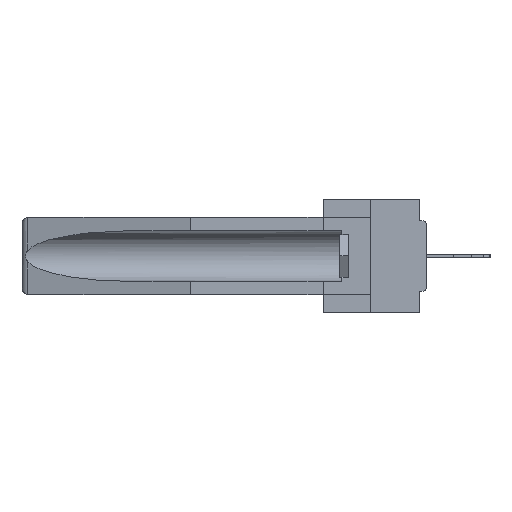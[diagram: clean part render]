
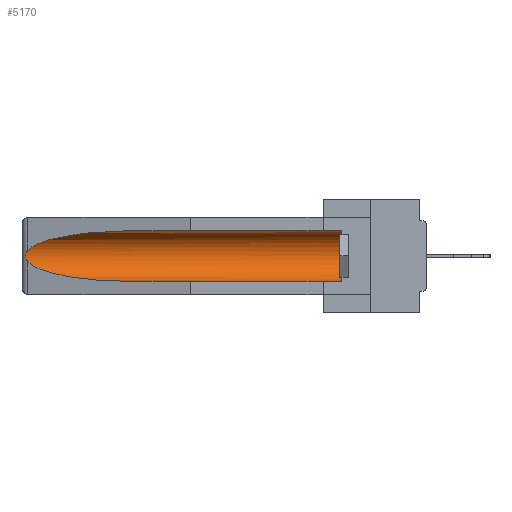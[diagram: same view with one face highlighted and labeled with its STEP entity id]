
A CAD part, left-side view. The second image highlights one B-rep face of the part: STEP entity #5170.
In plain terms, the highlighted cylindrical face has radius 2.857 mm (diameter 5.715 mm), a partial arc.
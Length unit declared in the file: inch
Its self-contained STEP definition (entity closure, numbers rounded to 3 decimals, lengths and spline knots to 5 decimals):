
#33 = CARTESIAN_POINT ( 'NONE',  ( 0.26537, 1.52718, -0.14972 ) ) ;
#827 = CARTESIAN_POINT ( 'NONE',  ( 0.25451, 1.48313, -0.09465 ) ) ;
#1087 = CARTESIAN_POINT ( 'NONE',  ( 0.25451, 1.48313, -0.24835 ) ) ;
#1258 = CARTESIAN_POINT ( 'NONE',  ( 0.21114, 1.30732, -0.284 ) ) ;
#2369 = CARTESIAN_POINT ( 'NONE',  ( 0.26597, 1.5296, -0.19026 ) ) ;
#2373 = DIRECTION ( 'NONE',  ( 0., -1., 0. ) ) ;
#3196 = VERTEX_POINT ( 'NONE', #5881 ) ;
#3373 = CARTESIAN_POINT ( 'NONE',  ( 0.155, 0.126, -0.284 ) ) ;
#4518 = CYLINDRICAL_SURFACE ( 'NONE', #18941, 0.1125 ) ;
#4991 = CARTESIAN_POINT ( 'NONE',  ( 0.26654, 1.53092, -0.15636 ) ) ;
#5170 = ADVANCED_FACE ( 'NONE', ( #16245 ), #4518, .F. ) ;
#5672 = DIRECTION ( 'NONE',  ( 0., 1., 0. ) ) ;
#5881 = CARTESIAN_POINT ( 'NONE',  ( 0.155, 1.07973, -0.059 ) ) ;
#5895 = ORIENTED_EDGE ( 'NONE', *, *, #28926, .T. ) ;
#5898 = VERTEX_POINT ( 'NONE', #27135 ) ;
#5992 =( BOUNDED_CURVE ( )  B_SPLINE_CURVE ( 3, ( #6052, #1087, #1258, #17963 ),
 .UNSPECIFIED., .F., .F. ) 
 B_SPLINE_CURVE_WITH_KNOTS ( ( 4, 4 ),
 ( 0.1948, 1.5708 ),
 .UNSPECIFIED. ) 
 CURVE ( )  GEOMETRIC_REPRESENTATION_ITEM ( )  RATIONAL_B_SPLINE_CURVE ( ( 1., 0.848, 0.848, 1. ) ) 
 REPRESENTATION_ITEM ( '' )  );
#6052 = CARTESIAN_POINT ( 'NONE',  ( 0.26537, 1.52718, -0.19328 ) ) ;
#9015 = ORIENTED_EDGE ( 'NONE', *, *, #17161, .F. ) ;
#9299 = DIRECTION ( 'NONE',  ( 0., 0., 1. ) ) ;
#10265 = CARTESIAN_POINT ( 'NONE',  ( 0.155, 1.07973, -0.059 ) ) ;
#11340 = CARTESIAN_POINT ( 'NONE',  ( 0.26537, 1.52718, -0.19328 ) ) ;
#11506 = ORIENTED_EDGE ( 'NONE', *, *, #30200, .T. ) ;
#11618 = DIRECTION ( 'NONE',  ( 0., 1., 0. ) ) ;
#11754 = LINE ( 'NONE', #25484, #19758 ) ;
#13215 = CARTESIAN_POINT ( 'NONE',  ( 0.26537, 1.52718, -0.14972 ) ) ;
#13261 = ORIENTED_EDGE ( 'NONE', *, *, #29223, .T. ) ;
#13619 = AXIS2_PLACEMENT_3D ( 'NONE', #18753, #2373, #28295 ) ;
#14417 = CARTESIAN_POINT ( 'NONE',  ( 0.26537, 1.52718, -0.19328 ) ) ;
#14434 = CARTESIAN_POINT ( 'NONE',  ( 0.2675, 1.53308, -0.17534 ) ) ;
#14921 = CARTESIAN_POINT ( 'NONE',  ( 0.26537, 1.52718, -0.14972 ) ) ;
#15838 = ORIENTED_EDGE ( 'NONE', *, *, #17611, .T. ) ;
#16245 = FACE_OUTER_BOUND ( 'NONE', #21789, .T. ) ;
#16270 = CARTESIAN_POINT ( 'NONE',  ( 0.2675, 1.53308, -0.16763 ) ) ;
#16675 = DIRECTION ( 'NONE',  ( 0., 1., 0. ) ) ;
#16735 = VERTEX_POINT ( 'NONE', #3373 ) ;
#16794 = B_SPLINE_CURVE_WITH_KNOTS ( 'NONE', 3,
 ( #33, #26119, #4991, #30167, #16270, #14434, #23837, #21062, #2369, #11340 ),
 .UNSPECIFIED., .F., .F.,
 ( 4, 2, 2, 2, 4 ),
 ( 0., 0.00029, 0.00058, 0.00087, 0.00117 ),
 .UNSPECIFIED. ) ;
#17161 = EDGE_CURVE ( 'NONE', #16735, #29163, #24661, .T. ) ;
#17611 = EDGE_CURVE ( 'NONE', #3196, #22894, #25350, .T. ) ;
#17963 = CARTESIAN_POINT ( 'NONE',  ( 0.155, 1.07973, -0.284 ) ) ;
#18753 = CARTESIAN_POINT ( 'NONE',  ( 0.155, 0.126, -0.1715 ) ) ;
#18941 = AXIS2_PLACEMENT_3D ( 'NONE', #23363, #11618, #9299 ) ;
#19545 = CARTESIAN_POINT ( 'NONE',  ( 0.21114, 1.30732, -0.059 ) ) ;
#19588 = VERTEX_POINT ( 'NONE', #14417 ) ;
#19722 = CARTESIAN_POINT ( 'NONE',  ( 0.155, -0.30754, -0.284 ) ) ;
#19758 = VECTOR ( 'NONE', #16675, 39.37008 ) ;
#21034 = ORIENTED_EDGE ( 'NONE', *, *, #25927, .T. ) ;
#21062 = CARTESIAN_POINT ( 'NONE',  ( 0.26655, 1.53094, -0.18657 ) ) ;
#21789 = EDGE_LOOP ( 'NONE', ( #15838, #5895, #13261, #9015, #11506, #21034 ) ) ;
#22894 = VERTEX_POINT ( 'NONE', #13215 ) ;
#23363 = CARTESIAN_POINT ( 'NONE',  ( 0.155, -0.30754, -0.1715 ) ) ;
#23837 = CARTESIAN_POINT ( 'NONE',  ( 0.2673, 1.53269, -0.17917 ) ) ;
#24407 = VECTOR ( 'NONE', #5672, 39.37008 ) ;
#24661 = LINE ( 'NONE', #19722, #24407 ) ;
#25042 = CARTESIAN_POINT ( 'NONE',  ( 0.155, 1.07973, -0.284 ) ) ;
#25350 =( BOUNDED_CURVE ( )  B_SPLINE_CURVE ( 3, ( #10265, #19545, #827, #14921 ),
 .UNSPECIFIED., .F., .F. ) 
 B_SPLINE_CURVE_WITH_KNOTS ( ( 4, 4 ),
 ( 4.71239, 6.08839 ),
 .UNSPECIFIED. ) 
 CURVE ( )  GEOMETRIC_REPRESENTATION_ITEM ( )  RATIONAL_B_SPLINE_CURVE ( ( 1., 0.848, 0.848, 1. ) ) 
 REPRESENTATION_ITEM ( '' )  );
#25484 = CARTESIAN_POINT ( 'NONE',  ( 0.155, -0.30754, -0.059 ) ) ;
#25927 = EDGE_CURVE ( 'NONE', #5898, #3196, #11754, .T. ) ;
#26119 = CARTESIAN_POINT ( 'NONE',  ( 0.26597, 1.52961, -0.15275 ) ) ;
#27135 = CARTESIAN_POINT ( 'NONE',  ( 0.155, 0.126, -0.059 ) ) ;
#28295 = DIRECTION ( 'NONE',  ( 0., 0., 1. ) ) ;
#28926 = EDGE_CURVE ( 'NONE', #22894, #19588, #16794, .T. ) ;
#29163 = VERTEX_POINT ( 'NONE', #25042 ) ;
#29223 = EDGE_CURVE ( 'NONE', #19588, #29163, #5992, .T. ) ;
#29828 = CIRCLE ( 'NONE', #13619, 0.1125 ) ;
#30167 = CARTESIAN_POINT ( 'NONE',  ( 0.2673, 1.5327, -0.16383 ) ) ;
#30200 = EDGE_CURVE ( 'NONE', #16735, #5898, #29828, .T. ) ;
